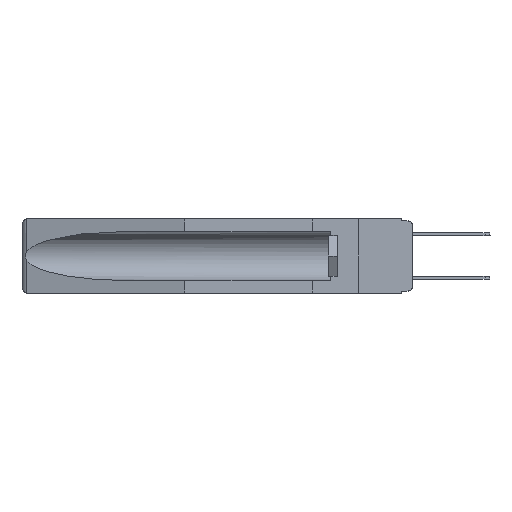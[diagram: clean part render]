
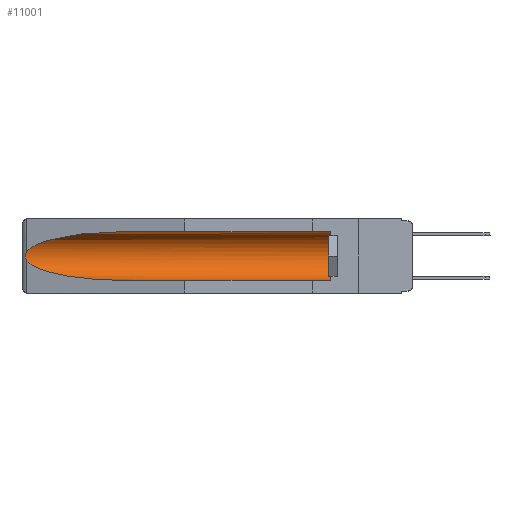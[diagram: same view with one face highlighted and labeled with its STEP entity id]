
A CAD part, left-side view. The second image highlights one B-rep face of the part: STEP entity #11001.
In plain terms, the highlighted cylindrical face has radius 2.857 mm (diameter 5.715 mm), a partial arc.
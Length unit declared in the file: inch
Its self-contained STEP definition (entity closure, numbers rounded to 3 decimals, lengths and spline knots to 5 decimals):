
#324 = CARTESIAN_POINT ( 'NONE',  ( 0.26597, 1.52961, -0.15275 ) ) ;
#432 = CARTESIAN_POINT ( 'NONE',  ( 0.2675, 1.53308, -0.16763 ) ) ;
#451 = CARTESIAN_POINT ( 'NONE',  ( 0.155, -0.30754, -0.059 ) ) ;
#458 = CARTESIAN_POINT ( 'NONE',  ( 0.26537, 1.52718, -0.19328 ) ) ;
#689 = DIRECTION ( 'NONE',  ( 0., 1., 0. ) ) ;
#1656 = CARTESIAN_POINT ( 'NONE',  ( 0.26537, 1.52718, -0.19328 ) ) ;
#1885 = VERTEX_POINT ( 'NONE', #12760 ) ;
#2596 = CARTESIAN_POINT ( 'NONE',  ( 0.2675, 1.53308, -0.17534 ) ) ;
#2767 = ORIENTED_EDGE ( 'NONE', *, *, #14195, .T. ) ;
#2998 = DIRECTION ( 'NONE',  ( 0., -1., 0. ) ) ;
#3234 = EDGE_CURVE ( 'NONE', #1885, #10861, #12954, .T. ) ;
#3727 = B_SPLINE_CURVE_WITH_KNOTS ( 'NONE', 3,
 ( #20837, #324, #5479, #15777, #432, #2596, #4267, #11102, #17933, #458 ),
 .UNSPECIFIED., .F., .F.,
 ( 4, 2, 2, 2, 4 ),
 ( 0., 0.00029, 0.00058, 0.00087, 0.00117 ),
 .UNSPECIFIED. ) ;
#4267 = CARTESIAN_POINT ( 'NONE',  ( 0.2673, 1.53269, -0.17917 ) ) ;
#4351 = CARTESIAN_POINT ( 'NONE',  ( 0.155, 0.126, -0.284 ) ) ;
#4851 =( BOUNDED_CURVE ( )  B_SPLINE_CURVE ( 3, ( #10906, #5634, #17524, #7321 ),
 .UNSPECIFIED., .F., .T. ) 
 B_SPLINE_CURVE_WITH_KNOTS ( ( 4, 4 ),
 ( 0.1948, 1.5708 ),
 .UNSPECIFIED. ) 
 CURVE ( )  GEOMETRIC_REPRESENTATION_ITEM ( )  RATIONAL_B_SPLINE_CURVE ( ( 1., 0.848, 0.848, 1. ) ) 
 REPRESENTATION_ITEM ( '' )  );
#4912 = VECTOR ( 'NONE', #689, 39.37008 ) ;
#5075 = VECTOR ( 'NONE', #7422, 39.37008 ) ;
#5206 = CARTESIAN_POINT ( 'NONE',  ( 0.155, -0.30754, -0.284 ) ) ;
#5479 = CARTESIAN_POINT ( 'NONE',  ( 0.26654, 1.53092, -0.15636 ) ) ;
#5634 = CARTESIAN_POINT ( 'NONE',  ( 0.25451, 1.48313, -0.24835 ) ) ;
#5840 = CYLINDRICAL_SURFACE ( 'NONE', #5985, 0.1125 ) ;
#5985 = AXIS2_PLACEMENT_3D ( 'NONE', #17723, #9313, #7309 ) ;
#6489 = CARTESIAN_POINT ( 'NONE',  ( 0.26537, 1.52718, -0.14972 ) ) ;
#7284 = CARTESIAN_POINT ( 'NONE',  ( 0.155, 1.07973, -0.059 ) ) ;
#7309 = DIRECTION ( 'NONE',  ( 0., 0., 1. ) ) ;
#7321 = CARTESIAN_POINT ( 'NONE',  ( 0.155, 1.07973, -0.284 ) ) ;
#7422 = DIRECTION ( 'NONE',  ( 0., 1., 0. ) ) ;
#7922 = ORIENTED_EDGE ( 'NONE', *, *, #17915, .T. ) ;
#8006 = ORIENTED_EDGE ( 'NONE', *, *, #10976, .F. ) ;
#8188 = ORIENTED_EDGE ( 'NONE', *, *, #9392, .T. ) ;
#8443 = VERTEX_POINT ( 'NONE', #6489 ) ;
#8454 = CARTESIAN_POINT ( 'NONE',  ( 0.26537, 1.52718, -0.14972 ) ) ;
#9094 = LINE ( 'NONE', #5206, #4912 ) ;
#9313 = DIRECTION ( 'NONE',  ( 0., 1., 0. ) ) ;
#9392 = EDGE_CURVE ( 'NONE', #10861, #8443, #18606, .T. ) ;
#9826 = DIRECTION ( 'NONE',  ( 0., 0., 1. ) ) ;
#10058 = VERTEX_POINT ( 'NONE', #1656 ) ;
#10861 = VERTEX_POINT ( 'NONE', #7284 ) ;
#10906 = CARTESIAN_POINT ( 'NONE',  ( 0.26537, 1.52718, -0.19328 ) ) ;
#10968 = EDGE_CURVE ( 'NONE', #8443, #10058, #3727, .T. ) ;
#10976 = EDGE_CURVE ( 'NONE', #20274, #16000, #9094, .T. ) ;
#11001 = ADVANCED_FACE ( 'NONE', ( #19407 ), #5840, .F. ) ;
#11102 = CARTESIAN_POINT ( 'NONE',  ( 0.26655, 1.53094, -0.18657 ) ) ;
#12012 = CARTESIAN_POINT ( 'NONE',  ( 0.25451, 1.48313, -0.09465 ) ) ;
#12760 = CARTESIAN_POINT ( 'NONE',  ( 0.155, 0.126, -0.059 ) ) ;
#12954 = LINE ( 'NONE', #451, #5075 ) ;
#13299 = AXIS2_PLACEMENT_3D ( 'NONE', #18342, #2998, #9826 ) ;
#14195 = EDGE_CURVE ( 'NONE', #10058, #16000, #4851, .T. ) ;
#15777 = CARTESIAN_POINT ( 'NONE',  ( 0.2673, 1.5327, -0.16383 ) ) ;
#16000 = VERTEX_POINT ( 'NONE', #19047 ) ;
#16534 = CIRCLE ( 'NONE', #13299, 0.1125 ) ;
#17300 = CARTESIAN_POINT ( 'NONE',  ( 0.21114, 1.30732, -0.059 ) ) ;
#17524 = CARTESIAN_POINT ( 'NONE',  ( 0.21114, 1.30732, -0.284 ) ) ;
#17723 = CARTESIAN_POINT ( 'NONE',  ( 0.155, -0.30754, -0.1715 ) ) ;
#17744 = ORIENTED_EDGE ( 'NONE', *, *, #3234, .T. ) ;
#17915 = EDGE_CURVE ( 'NONE', #20274, #1885, #16534, .T. ) ;
#17933 = CARTESIAN_POINT ( 'NONE',  ( 0.26597, 1.5296, -0.19026 ) ) ;
#18342 = CARTESIAN_POINT ( 'NONE',  ( 0.155, 0.126, -0.1715 ) ) ;
#18606 =( BOUNDED_CURVE ( )  B_SPLINE_CURVE ( 3, ( #20662, #17300, #12012, #8454 ),
 .UNSPECIFIED., .F., .T. ) 
 B_SPLINE_CURVE_WITH_KNOTS ( ( 4, 4 ),
 ( 4.71239, 6.08839 ),
 .UNSPECIFIED. ) 
 CURVE ( )  GEOMETRIC_REPRESENTATION_ITEM ( )  RATIONAL_B_SPLINE_CURVE ( ( 1., 0.848, 0.848, 1. ) ) 
 REPRESENTATION_ITEM ( '' )  );
#18610 = EDGE_LOOP ( 'NONE', ( #8188, #21881, #2767, #8006, #7922, #17744 ) ) ;
#19047 = CARTESIAN_POINT ( 'NONE',  ( 0.155, 1.07973, -0.284 ) ) ;
#19407 = FACE_OUTER_BOUND ( 'NONE', #18610, .T. ) ;
#20274 = VERTEX_POINT ( 'NONE', #4351 ) ;
#20662 = CARTESIAN_POINT ( 'NONE',  ( 0.155, 1.07973, -0.059 ) ) ;
#20837 = CARTESIAN_POINT ( 'NONE',  ( 0.26537, 1.52718, -0.14972 ) ) ;
#21881 = ORIENTED_EDGE ( 'NONE', *, *, #10968, .T. ) ;
